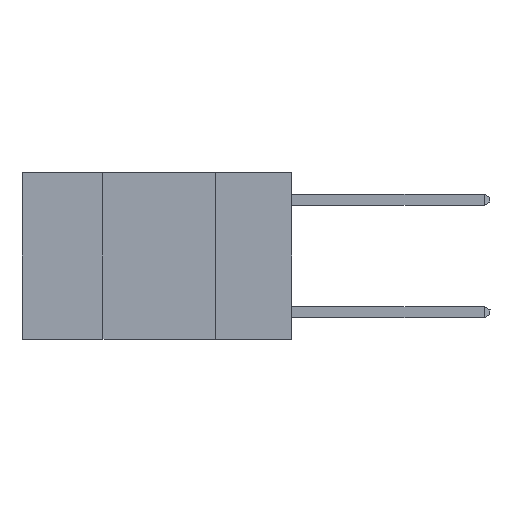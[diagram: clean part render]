
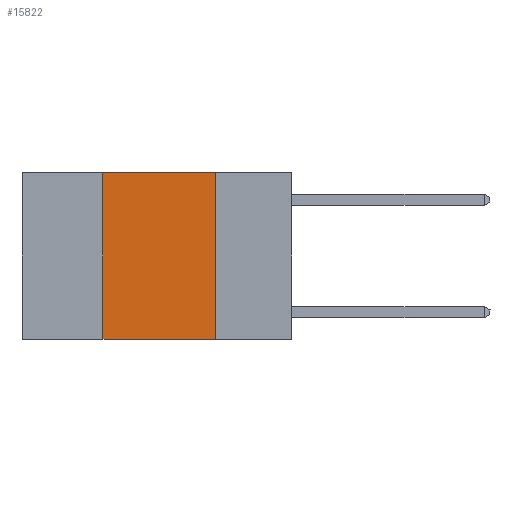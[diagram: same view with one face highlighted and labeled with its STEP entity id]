
A CAD part, left-side view. The second image highlights one B-rep face of the part: STEP entity #15822.
In plain terms, the highlighted planar face has unit normal (-1, 0, 0).
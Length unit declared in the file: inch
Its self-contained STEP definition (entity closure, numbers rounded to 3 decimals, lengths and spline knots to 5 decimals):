
#228 = DIRECTION ( 'NONE',  ( 0., 0., -1. ) ) ;
#685 = CARTESIAN_POINT ( 'NONE',  ( 0., 0.42, -0.37 ) ) ;
#1526 = EDGE_CURVE ( 'NONE', #25191, #17363, #7858, .T. ) ;
#2049 = ORIENTED_EDGE ( 'NONE', *, *, #19517, .T. ) ;
#2317 = VECTOR ( 'NONE', #14886, 39.37008 ) ;
#3283 = CARTESIAN_POINT ( 'NONE',  ( 0., 0.17, 0. ) ) ;
#3348 = CARTESIAN_POINT ( 'NONE',  ( 0., 0.17, 0. ) ) ;
#4449 = LINE ( 'NONE', #19990, #26163 ) ;
#5238 = ORIENTED_EDGE ( 'NONE', *, *, #10841, .F. ) ;
#5329 = FACE_OUTER_BOUND ( 'NONE', #9817, .T. ) ;
#6418 = ORIENTED_EDGE ( 'NONE', *, *, #6444, .F. ) ;
#6444 = EDGE_CURVE ( 'NONE', #8304, #9383, #24959, .T. ) ;
#7015 = ORIENTED_EDGE ( 'NONE', *, *, #1526, .F. ) ;
#7858 = LINE ( 'NONE', #3283, #23913 ) ;
#8304 = VERTEX_POINT ( 'NONE', #685 ) ;
#9383 = VERTEX_POINT ( 'NONE', #26722 ) ;
#9817 = EDGE_LOOP ( 'NONE', ( #7015, #5238, #6418, #2049 ) ) ;
#10511 = PLANE ( 'NONE',  #11300 ) ;
#10841 = EDGE_CURVE ( 'NONE', #9383, #25191, #25363, .T. ) ;
#11300 = AXIS2_PLACEMENT_3D ( 'NONE', #25099, #12663, #228 ) ;
#12663 = DIRECTION ( 'NONE',  ( 1., 0., 0. ) ) ;
#12711 = CARTESIAN_POINT ( 'NONE',  ( 0., 0.6, 0. ) ) ;
#14886 = DIRECTION ( 'NONE',  ( 0., -1., 0. ) ) ;
#15822 = ADVANCED_FACE ( 'NONE', ( #5329 ), #10511, .F. ) ;
#17363 = VERTEX_POINT ( 'NONE', #24069 ) ;
#19517 = EDGE_CURVE ( 'NONE', #8304, #17363, #4449, .T. ) ;
#19990 = CARTESIAN_POINT ( 'NONE',  ( 0., 0.6, -0.37 ) ) ;
#23913 = VECTOR ( 'NONE', #24317, 39.37008 ) ;
#24069 = CARTESIAN_POINT ( 'NONE',  ( 0., 0.17, -0.37 ) ) ;
#24317 = DIRECTION ( 'NONE',  ( 0., 0., -1. ) ) ;
#24342 = VECTOR ( 'NONE', #26972, 39.37008 ) ;
#24934 = CARTESIAN_POINT ( 'NONE',  ( 0., 0.42, 0. ) ) ;
#24959 = LINE ( 'NONE', #24934, #24342 ) ;
#25099 = CARTESIAN_POINT ( 'NONE',  ( 0., 0.6, 0. ) ) ;
#25191 = VERTEX_POINT ( 'NONE', #3348 ) ;
#25363 = LINE ( 'NONE', #12711, #2317 ) ;
#26163 = VECTOR ( 'NONE', #26214, 39.37008 ) ;
#26214 = DIRECTION ( 'NONE',  ( 0., -1., 0. ) ) ;
#26722 = CARTESIAN_POINT ( 'NONE',  ( 0., 0.42, 0. ) ) ;
#26972 = DIRECTION ( 'NONE',  ( 0., 0., 1. ) ) ;
